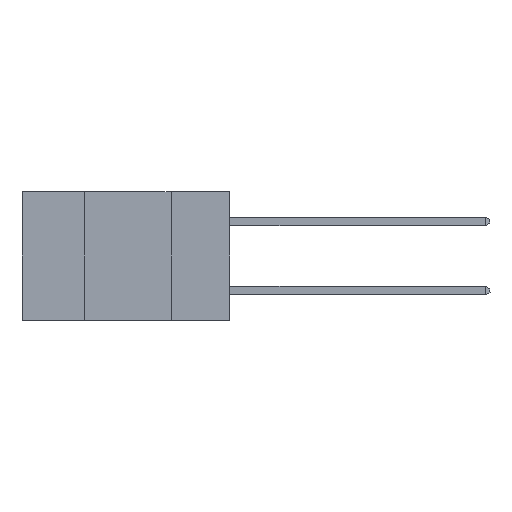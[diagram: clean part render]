
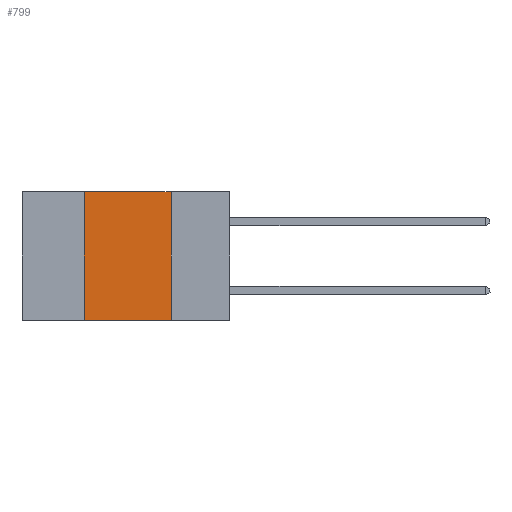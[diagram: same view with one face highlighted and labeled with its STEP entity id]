
A CAD part, left-side view. The second image highlights one B-rep face of the part: STEP entity #799.
In plain terms, the highlighted planar face has unit normal (-1, 0, 0).
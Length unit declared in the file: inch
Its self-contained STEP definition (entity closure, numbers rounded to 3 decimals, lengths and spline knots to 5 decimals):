
#128 = CARTESIAN_POINT ( 'NONE',  ( 0., 0.17, 0. ) ) ;
#516 = CARTESIAN_POINT ( 'NONE',  ( 0., 0.17, 0. ) ) ;
#673 = EDGE_CURVE ( 'NONE', #22970, #20303, #3257, .T. ) ;
#799 = ADVANCED_FACE ( 'NONE', ( #3295 ), #9024, .F. ) ;
#1544 = LINE ( 'NONE', #30304, #5926 ) ;
#3153 = LINE ( 'NONE', #128, #19328 ) ;
#3179 = VERTEX_POINT ( 'NONE', #4571 ) ;
#3257 = LINE ( 'NONE', #7542, #23585 ) ;
#3295 = FACE_OUTER_BOUND ( 'NONE', #9058, .T. ) ;
#4571 = CARTESIAN_POINT ( 'NONE',  ( 0., 0.42, 0. ) ) ;
#5926 = VECTOR ( 'NONE', #27907, 39.37008 ) ;
#7114 = CARTESIAN_POINT ( 'NONE',  ( 0., 0.6, 0. ) ) ;
#7542 = CARTESIAN_POINT ( 'NONE',  ( 0., 0.6, -0.37 ) ) ;
#7846 = DIRECTION ( 'NONE',  ( 0., -1., 0. ) ) ;
#8224 = VERTEX_POINT ( 'NONE', #516 ) ;
#9024 = PLANE ( 'NONE',  #18513 ) ;
#9058 = EDGE_LOOP ( 'NONE', ( #13083, #17848, #9490, #25147 ) ) ;
#9089 = CARTESIAN_POINT ( 'NONE',  ( 0., 0.17, -0.37 ) ) ;
#9429 = DIRECTION ( 'NONE',  ( 0., 0., 1. ) ) ;
#9490 = ORIENTED_EDGE ( 'NONE', *, *, #19689, .F. ) ;
#9805 = VECTOR ( 'NONE', #9429, 39.37008 ) ;
#11377 = DIRECTION ( 'NONE',  ( 0., 0., -1. ) ) ;
#11688 = DIRECTION ( 'NONE',  ( 1., 0., 0. ) ) ;
#13083 = ORIENTED_EDGE ( 'NONE', *, *, #21576, .F. ) ;
#13877 = CARTESIAN_POINT ( 'NONE',  ( 0., 0.42, -0.37 ) ) ;
#17848 = ORIENTED_EDGE ( 'NONE', *, *, #18145, .F. ) ;
#18145 = EDGE_CURVE ( 'NONE', #3179, #8224, #1544, .T. ) ;
#18513 = AXIS2_PLACEMENT_3D ( 'NONE', #7114, #11688, #11377 ) ;
#19328 = VECTOR ( 'NONE', #21484, 39.37008 ) ;
#19689 = EDGE_CURVE ( 'NONE', #22970, #3179, #29867, .T. ) ;
#20303 = VERTEX_POINT ( 'NONE', #9089 ) ;
#21275 = CARTESIAN_POINT ( 'NONE',  ( 0., 0.42, 0. ) ) ;
#21484 = DIRECTION ( 'NONE',  ( 0., 0., -1. ) ) ;
#21576 = EDGE_CURVE ( 'NONE', #8224, #20303, #3153, .T. ) ;
#22970 = VERTEX_POINT ( 'NONE', #13877 ) ;
#23585 = VECTOR ( 'NONE', #7846, 39.37008 ) ;
#25147 = ORIENTED_EDGE ( 'NONE', *, *, #673, .T. ) ;
#27907 = DIRECTION ( 'NONE',  ( 0., -1., 0. ) ) ;
#29867 = LINE ( 'NONE', #21275, #9805 ) ;
#30304 = CARTESIAN_POINT ( 'NONE',  ( 0., 0.6, 0. ) ) ;
